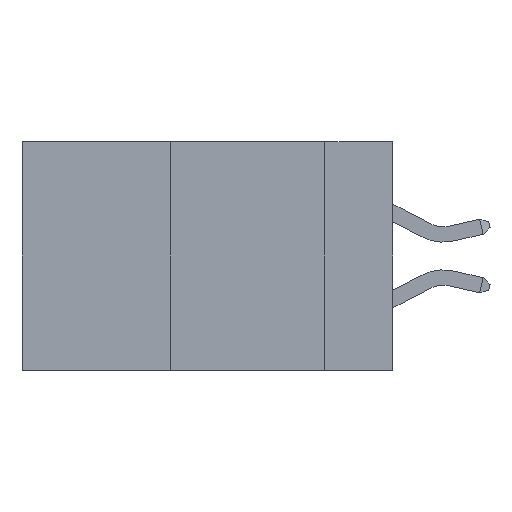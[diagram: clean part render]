
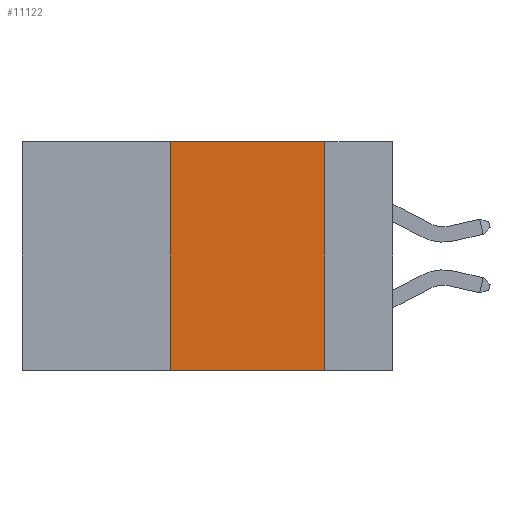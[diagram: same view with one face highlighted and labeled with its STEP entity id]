
A CAD part, left-side view. The second image highlights one B-rep face of the part: STEP entity #11122.
In plain terms, the highlighted planar face has unit normal (-1, 0, 0).
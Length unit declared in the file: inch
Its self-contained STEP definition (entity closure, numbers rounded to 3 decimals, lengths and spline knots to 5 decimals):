
#559 = CARTESIAN_POINT ( 'NONE',  ( 0., 0.6, 0. ) ) ;
#2608 = CARTESIAN_POINT ( 'NONE',  ( 0., 0.36, -0.37 ) ) ;
#5468 = CARTESIAN_POINT ( 'NONE',  ( 0., 0.6, 0. ) ) ;
#5575 = VERTEX_POINT ( 'NONE', #19178 ) ;
#7253 = EDGE_CURVE ( 'NONE', #5575, #7786, #10803, .T. ) ;
#7786 = VERTEX_POINT ( 'NONE', #20889 ) ;
#10803 = LINE ( 'NONE', #12282, #11766 ) ;
#11122 = ADVANCED_FACE ( 'NONE', ( #11344 ), #36669, .F. ) ;
#11344 = FACE_OUTER_BOUND ( 'NONE', #20495, .T. ) ;
#11766 = VECTOR ( 'NONE', #26340, 39.37008 ) ;
#12282 = CARTESIAN_POINT ( 'NONE',  ( 0., 0.11, 0. ) ) ;
#12883 = CARTESIAN_POINT ( 'NONE',  ( 0., 0.36, 0. ) ) ;
#15137 = CARTESIAN_POINT ( 'NONE',  ( 0., 0.36, 0. ) ) ;
#15806 = DIRECTION ( 'NONE',  ( 1., 0., 0. ) ) ;
#19178 = CARTESIAN_POINT ( 'NONE',  ( 0., 0.11, 0. ) ) ;
#19983 = EDGE_CURVE ( 'NONE', #21823, #7786, #25760, .T. ) ;
#20495 = EDGE_LOOP ( 'NONE', ( #37724, #23066, #27230, #25284 ) ) ;
#20889 = CARTESIAN_POINT ( 'NONE',  ( 0., 0.11, -0.37 ) ) ;
#21823 = VERTEX_POINT ( 'NONE', #2608 ) ;
#22475 = AXIS2_PLACEMENT_3D ( 'NONE', #559, #15806, #36933 ) ;
#23066 = ORIENTED_EDGE ( 'NONE', *, *, #32864, .F. ) ;
#23571 = CARTESIAN_POINT ( 'NONE',  ( 0., 0.6, -0.37 ) ) ;
#24750 = EDGE_CURVE ( 'NONE', #21823, #36155, #30986, .T. ) ;
#25284 = ORIENTED_EDGE ( 'NONE', *, *, #19983, .T. ) ;
#25433 = LINE ( 'NONE', #5468, #33027 ) ;
#25760 = LINE ( 'NONE', #23571, #38513 ) ;
#25787 = VECTOR ( 'NONE', #30638, 39.37008 ) ;
#26340 = DIRECTION ( 'NONE',  ( 0., 0., -1. ) ) ;
#26631 = DIRECTION ( 'NONE',  ( 0., -1., 0. ) ) ;
#27230 = ORIENTED_EDGE ( 'NONE', *, *, #24750, .F. ) ;
#30638 = DIRECTION ( 'NONE',  ( 0., 0., 1. ) ) ;
#30986 = LINE ( 'NONE', #12883, #25787 ) ;
#32771 = DIRECTION ( 'NONE',  ( 0., -1., 0. ) ) ;
#32864 = EDGE_CURVE ( 'NONE', #36155, #5575, #25433, .T. ) ;
#33027 = VECTOR ( 'NONE', #32771, 39.37008 ) ;
#36155 = VERTEX_POINT ( 'NONE', #15137 ) ;
#36669 = PLANE ( 'NONE',  #22475 ) ;
#36933 = DIRECTION ( 'NONE',  ( 0., 0., -1. ) ) ;
#37724 = ORIENTED_EDGE ( 'NONE', *, *, #7253, .F. ) ;
#38513 = VECTOR ( 'NONE', #26631, 39.37008 ) ;
